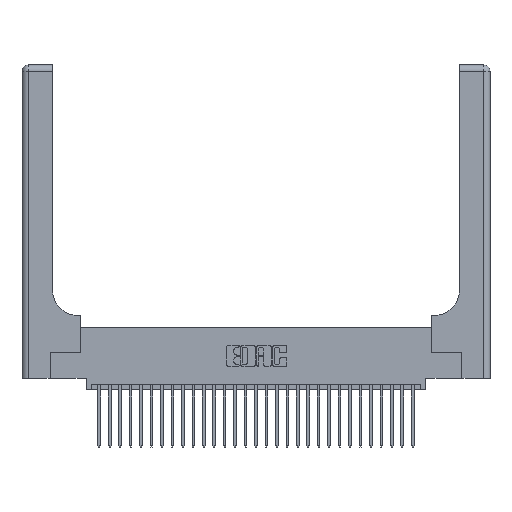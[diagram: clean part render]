
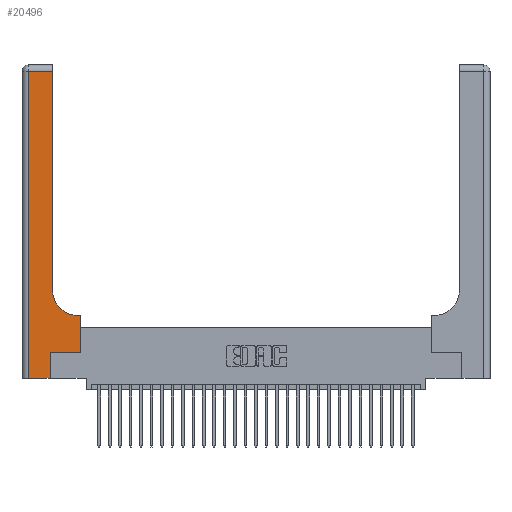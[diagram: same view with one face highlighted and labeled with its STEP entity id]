
A CAD part, top view. The second image highlights one B-rep face of the part: STEP entity #20496.
In plain terms, the highlighted planar face has unit normal (0, 0, 1).
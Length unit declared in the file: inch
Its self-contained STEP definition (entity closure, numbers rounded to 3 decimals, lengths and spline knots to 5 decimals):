
#614 = ORIENTED_EDGE ( 'NONE', *, *, #28790, .T. ) ;
#1258 = CARTESIAN_POINT ( 'NONE',  ( 0.5585, 0.25, 0.37 ) ) ;
#1869 = EDGE_CURVE ( 'NONE', #6967, #28511, #30711, .T. ) ;
#2018 = VECTOR ( 'NONE', #29925, 39.37008 ) ;
#2151 = CARTESIAN_POINT ( 'NONE',  ( 0.06, 3., 0.37 ) ) ;
#2950 = ORIENTED_EDGE ( 'NONE', *, *, #27061, .T. ) ;
#3399 = DIRECTION ( 'NONE',  ( 0., 0., -1. ) ) ;
#4261 = VERTEX_POINT ( 'NONE', #27560 ) ;
#4824 = ORIENTED_EDGE ( 'NONE', *, *, #25524, .T. ) ;
#5059 = VECTOR ( 'NONE', #23885, 39.37008 ) ;
#5069 = DIRECTION ( 'NONE',  ( 0., 0., -1. ) ) ;
#5243 = VECTOR ( 'NONE', #14856, 39.37008 ) ;
#6030 = DIRECTION ( 'NONE',  ( 1., 0., 0. ) ) ;
#6490 = EDGE_CURVE ( 'NONE', #9935, #23371, #8411, .T. ) ;
#6546 = FACE_OUTER_BOUND ( 'NONE', #22620, .T. ) ;
#6754 = EDGE_CURVE ( 'NONE', #7615, #11099, #7257, .T. ) ;
#6967 = VERTEX_POINT ( 'NONE', #22157 ) ;
#7257 = LINE ( 'NONE', #21438, #25694 ) ;
#7466 = ORIENTED_EDGE ( 'NONE', *, *, #6754, .T. ) ;
#7615 = VERTEX_POINT ( 'NONE', #20055 ) ;
#7992 = VECTOR ( 'NONE', #21287, 39.37008 ) ;
#8351 = LINE ( 'NONE', #27599, #20471 ) ;
#8411 = LINE ( 'NONE', #1258, #21986 ) ;
#8452 = VECTOR ( 'NONE', #15111, 39.37008 ) ;
#8484 = LINE ( 'NONE', #27559, #2018 ) ;
#8542 = CARTESIAN_POINT ( 'NONE',  ( 0.5415, 0.6, 0.37 ) ) ;
#8985 = ORIENTED_EDGE ( 'NONE', *, *, #6490, .T. ) ;
#9935 = VERTEX_POINT ( 'NONE', #19275 ) ;
#11099 = VERTEX_POINT ( 'NONE', #27731 ) ;
#12195 = LINE ( 'NONE', #2151, #5059 ) ;
#12793 = ORIENTED_EDGE ( 'NONE', *, *, #1869, .T. ) ;
#13011 = PLANE ( 'NONE',  #15623 ) ;
#14150 = LINE ( 'NONE', #24693, #8452 ) ;
#14466 = LINE ( 'NONE', #18923, #7992 ) ;
#14582 = EDGE_CURVE ( 'NONE', #23371, #24387, #14466, .T. ) ;
#14856 = DIRECTION ( 'NONE',  ( -1., 0., 0. ) ) ;
#15111 = DIRECTION ( 'NONE',  ( 1., 0., 0. ) ) ;
#15623 = AXIS2_PLACEMENT_3D ( 'NONE', #24963, #3399, #20288 ) ;
#15925 = CARTESIAN_POINT ( 'NONE',  ( 0.2915, 0.85, 0.37 ) ) ;
#16994 = ORIENTED_EDGE ( 'NONE', *, *, #14582, .T. ) ;
#17203 = CARTESIAN_POINT ( 'NONE',  ( 0., 2.94, 0.37 ) ) ;
#17357 = AXIS2_PLACEMENT_3D ( 'NONE', #19536, #5069, #21913 ) ;
#18170 = ORIENTED_EDGE ( 'NONE', *, *, #26018, .T. ) ;
#18277 = DIRECTION ( 'NONE',  ( 0., 1., 0. ) ) ;
#18923 = CARTESIAN_POINT ( 'NONE',  ( 0.2915, 0.6, 0.37 ) ) ;
#19275 = CARTESIAN_POINT ( 'NONE',  ( 0.5585, 0.25, 0.37 ) ) ;
#19536 = CARTESIAN_POINT ( 'NONE',  ( 0.5415, 0.85, 0.37 ) ) ;
#20055 = CARTESIAN_POINT ( 'NONE',  ( 0.269, 0., 0.37 ) ) ;
#20288 = DIRECTION ( 'NONE',  ( -1., 0., 0. ) ) ;
#20471 = VECTOR ( 'NONE', #6030, 39.37008 ) ;
#20496 = ADVANCED_FACE ( 'NONE', ( #6546 ), #13011, .F. ) ;
#21158 = EDGE_CURVE ( 'NONE', #11099, #9935, #8351, .T. ) ;
#21287 = DIRECTION ( 'NONE',  ( -1., 0., 0. ) ) ;
#21438 = CARTESIAN_POINT ( 'NONE',  ( 0.269, 0., 0.37 ) ) ;
#21913 = DIRECTION ( 'NONE',  ( 1., 0., 0. ) ) ;
#21986 = VECTOR ( 'NONE', #18277, 39.37008 ) ;
#22157 = CARTESIAN_POINT ( 'NONE',  ( 0.2915, 2.94, 0.37 ) ) ;
#22269 = CARTESIAN_POINT ( 'NONE',  ( 0.06, 2.94, 0.37 ) ) ;
#22620 = EDGE_LOOP ( 'NONE', ( #4824, #12793, #2950, #18170, #7466, #27375, #8985, #16994, #614 ) ) ;
#23371 = VERTEX_POINT ( 'NONE', #30675 ) ;
#23819 = DIRECTION ( 'NONE',  ( 0., 1., 0. ) ) ;
#23885 = DIRECTION ( 'NONE',  ( 0., -1., 0. ) ) ;
#24387 = VERTEX_POINT ( 'NONE', #8542 ) ;
#24693 = CARTESIAN_POINT ( 'NONE',  ( 0., 0., 0.37 ) ) ;
#24963 = CARTESIAN_POINT ( 'NONE',  ( 0., 3., 0.37 ) ) ;
#25524 = EDGE_CURVE ( 'NONE', #30336, #6967, #8484, .T. ) ;
#25694 = VECTOR ( 'NONE', #23819, 39.37008 ) ;
#26018 = EDGE_CURVE ( 'NONE', #4261, #7615, #14150, .T. ) ;
#27061 = EDGE_CURVE ( 'NONE', #28511, #4261, #12195, .T. ) ;
#27375 = ORIENTED_EDGE ( 'NONE', *, *, #21158, .T. ) ;
#27559 = CARTESIAN_POINT ( 'NONE',  ( 0.2915, 3., 0.37 ) ) ;
#27560 = CARTESIAN_POINT ( 'NONE',  ( 0.06, 0., 0.37 ) ) ;
#27599 = CARTESIAN_POINT ( 'NONE',  ( 0.269, 0.25, 0.37 ) ) ;
#27731 = CARTESIAN_POINT ( 'NONE',  ( 0.269, 0.25, 0.37 ) ) ;
#27922 = CIRCLE ( 'NONE', #17357, 0.25 ) ;
#28511 = VERTEX_POINT ( 'NONE', #22269 ) ;
#28790 = EDGE_CURVE ( 'NONE', #24387, #30336, #27922, .T. ) ;
#29925 = DIRECTION ( 'NONE',  ( 0., 1., 0. ) ) ;
#30336 = VERTEX_POINT ( 'NONE', #15925 ) ;
#30675 = CARTESIAN_POINT ( 'NONE',  ( 0.5585, 0.6, 0.37 ) ) ;
#30711 = LINE ( 'NONE', #17203, #5243 ) ;
